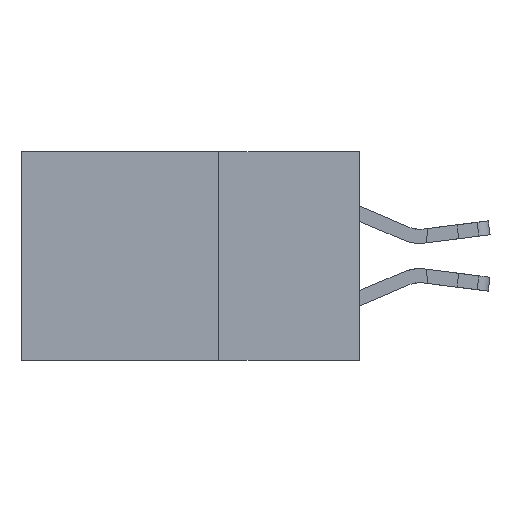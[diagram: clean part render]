
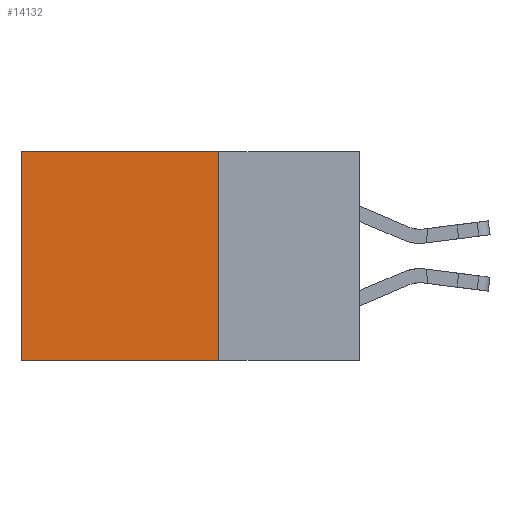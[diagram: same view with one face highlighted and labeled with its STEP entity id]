
A CAD part, left-side view. The second image highlights one B-rep face of the part: STEP entity #14132.
In plain terms, the highlighted planar face has unit normal (-1, 0, 0).
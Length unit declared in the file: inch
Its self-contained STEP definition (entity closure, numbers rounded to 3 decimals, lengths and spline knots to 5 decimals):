
#226 = CARTESIAN_POINT ( 'NONE',  ( 0.2875, 0.25, -0.37 ) ) ;
#2288 = ORIENTED_EDGE ( 'NONE', *, *, #15526, .T. ) ;
#2309 = EDGE_CURVE ( 'NONE', #12142, #8881, #20077, .T. ) ;
#2989 = LINE ( 'NONE', #19990, #16017 ) ;
#5124 = DIRECTION ( 'NONE',  ( 0., 1., 0. ) ) ;
#5451 = DIRECTION ( 'NONE',  ( 1., 0., 0. ) ) ;
#5918 = FACE_OUTER_BOUND ( 'NONE', #21698, .T. ) ;
#5950 = EDGE_CURVE ( 'NONE', #12142, #21573, #26400, .T. ) ;
#6051 = CARTESIAN_POINT ( 'NONE',  ( 0.2875, 0.25, 0. ) ) ;
#7976 = PLANE ( 'NONE',  #27496 ) ;
#8772 = LINE ( 'NONE', #13660, #21345 ) ;
#8881 = VERTEX_POINT ( 'NONE', #226 ) ;
#9996 = VERTEX_POINT ( 'NONE', #22754 ) ;
#12041 = VECTOR ( 'NONE', #20236, 39.37008 ) ;
#12142 = VERTEX_POINT ( 'NONE', #29790 ) ;
#12970 = ORIENTED_EDGE ( 'NONE', *, *, #5950, .T. ) ;
#13660 = CARTESIAN_POINT ( 'NONE',  ( 0.2875, 0.25, -0.37 ) ) ;
#14132 = ADVANCED_FACE ( 'NONE', ( #5918 ), #7976, .F. ) ;
#14926 = CARTESIAN_POINT ( 'NONE',  ( 0.2875, 0.25, 0. ) ) ;
#15526 = EDGE_CURVE ( 'NONE', #21573, #9996, #2989, .T. ) ;
#16017 = VECTOR ( 'NONE', #24866, 39.37008 ) ;
#19990 = CARTESIAN_POINT ( 'NONE',  ( 0.2875, 0.6, 0. ) ) ;
#20077 = LINE ( 'NONE', #6051, #12041 ) ;
#20236 = DIRECTION ( 'NONE',  ( 0., 0., -1. ) ) ;
#20900 = DIRECTION ( 'NONE',  ( 0., 1., 0. ) ) ;
#21345 = VECTOR ( 'NONE', #20900, 39.37008 ) ;
#21573 = VERTEX_POINT ( 'NONE', #22642 ) ;
#21698 = EDGE_LOOP ( 'NONE', ( #2288, #25760, #29709, #12970 ) ) ;
#22068 = VECTOR ( 'NONE', #5124, 39.37008 ) ;
#22642 = CARTESIAN_POINT ( 'NONE',  ( 0.2875, 0.6, 0. ) ) ;
#22754 = CARTESIAN_POINT ( 'NONE',  ( 0.2875, 0.6, -0.37 ) ) ;
#24866 = DIRECTION ( 'NONE',  ( 0., 0., -1. ) ) ;
#25475 = EDGE_CURVE ( 'NONE', #8881, #9996, #8772, .T. ) ;
#25760 = ORIENTED_EDGE ( 'NONE', *, *, #25475, .F. ) ;
#26400 = LINE ( 'NONE', #26701, #22068 ) ;
#26701 = CARTESIAN_POINT ( 'NONE',  ( 0.2875, 0.25, 0. ) ) ;
#27496 = AXIS2_PLACEMENT_3D ( 'NONE', #14926, #5451, #29564 ) ;
#29564 = DIRECTION ( 'NONE',  ( 0., 0., -1. ) ) ;
#29709 = ORIENTED_EDGE ( 'NONE', *, *, #2309, .F. ) ;
#29790 = CARTESIAN_POINT ( 'NONE',  ( 0.2875, 0.25, 0. ) ) ;
